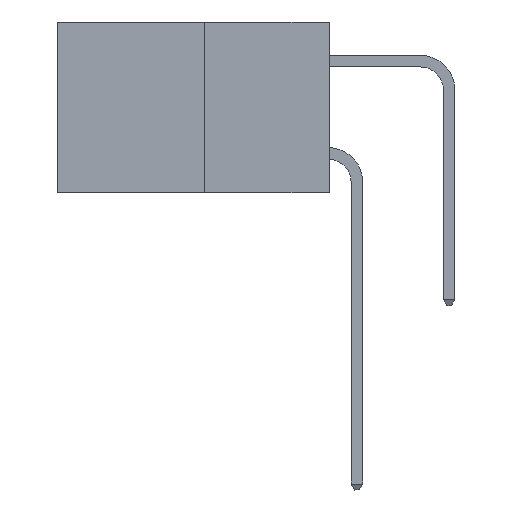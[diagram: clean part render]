
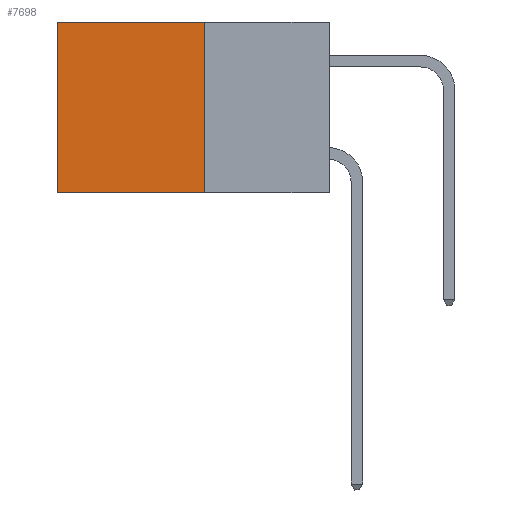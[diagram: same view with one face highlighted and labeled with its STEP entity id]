
A CAD part, left-side view. The second image highlights one B-rep face of the part: STEP entity #7698.
In plain terms, the highlighted planar face has unit normal (-1, 0, 0).
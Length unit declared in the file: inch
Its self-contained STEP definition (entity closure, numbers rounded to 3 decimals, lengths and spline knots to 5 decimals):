
#1098 = DIRECTION ( 'NONE',  ( 0., 0., -1. ) ) ;
#1212 = CARTESIAN_POINT ( 'NONE',  ( 0.277, 0.27, 0. ) ) ;
#2417 = DIRECTION ( 'NONE',  ( 0., 1., 0. ) ) ;
#3024 = DIRECTION ( 'NONE',  ( 0., 1., 0. ) ) ;
#3867 = VECTOR ( 'NONE', #3024, 39.37008 ) ;
#6634 = EDGE_LOOP ( 'NONE', ( #13667, #18719, #14979, #10973 ) ) ;
#7698 = ADVANCED_FACE ( 'NONE', ( #11900 ), #22567, .F. ) ;
#8327 = DIRECTION ( 'NONE',  ( 0., 0., -1. ) ) ;
#8357 = LINE ( 'NONE', #22467, #16808 ) ;
#9672 = CARTESIAN_POINT ( 'NONE',  ( 0.277, 0.27, -0.37 ) ) ;
#9927 = VERTEX_POINT ( 'NONE', #19689 ) ;
#10417 = CARTESIAN_POINT ( 'NONE',  ( 0.277, 0.27, 0. ) ) ;
#10973 = ORIENTED_EDGE ( 'NONE', *, *, #16075, .T. ) ;
#11900 = FACE_OUTER_BOUND ( 'NONE', #6634, .T. ) ;
#12034 = DIRECTION ( 'NONE',  ( 1., 0., 0. ) ) ;
#12122 = VECTOR ( 'NONE', #2417, 39.37008 ) ;
#12949 = EDGE_CURVE ( 'NONE', #19260, #16581, #17412, .T. ) ;
#13567 = LINE ( 'NONE', #1212, #3867 ) ;
#13667 = ORIENTED_EDGE ( 'NONE', *, *, #18273, .T. ) ;
#14780 = CARTESIAN_POINT ( 'NONE',  ( 0.277, 0.27, -0.37 ) ) ;
#14979 = ORIENTED_EDGE ( 'NONE', *, *, #22164, .F. ) ;
#15447 = VERTEX_POINT ( 'NONE', #10417 ) ;
#15528 = CARTESIAN_POINT ( 'NONE',  ( 0.277, 0.27, -0.37 ) ) ;
#16075 = EDGE_CURVE ( 'NONE', #15447, #9927, #13567, .T. ) ;
#16581 = VERTEX_POINT ( 'NONE', #20452 ) ;
#16808 = VECTOR ( 'NONE', #8327, 39.37008 ) ;
#17412 = LINE ( 'NONE', #9672, #12122 ) ;
#18044 = CARTESIAN_POINT ( 'NONE',  ( 0.277, 0.59, -0.37 ) ) ;
#18273 = EDGE_CURVE ( 'NONE', #9927, #16581, #20899, .T. ) ;
#18491 = AXIS2_PLACEMENT_3D ( 'NONE', #15528, #12034, #1098 ) ;
#18719 = ORIENTED_EDGE ( 'NONE', *, *, #12949, .F. ) ;
#19260 = VERTEX_POINT ( 'NONE', #14780 ) ;
#19689 = CARTESIAN_POINT ( 'NONE',  ( 0.277, 0.59, 0. ) ) ;
#19831 = VECTOR ( 'NONE', #19867, 39.37008 ) ;
#19867 = DIRECTION ( 'NONE',  ( 0., 0., -1. ) ) ;
#20452 = CARTESIAN_POINT ( 'NONE',  ( 0.277, 0.59, -0.37 ) ) ;
#20899 = LINE ( 'NONE', #18044, #19831 ) ;
#22164 = EDGE_CURVE ( 'NONE', #15447, #19260, #8357, .T. ) ;
#22467 = CARTESIAN_POINT ( 'NONE',  ( 0.277, 0.27, -0.37 ) ) ;
#22567 = PLANE ( 'NONE',  #18491 ) ;
